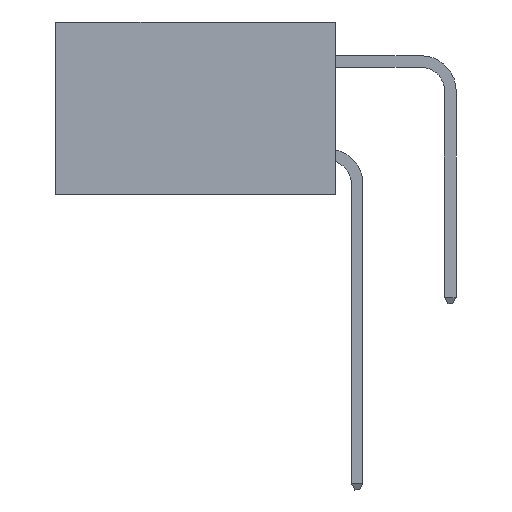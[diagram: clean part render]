
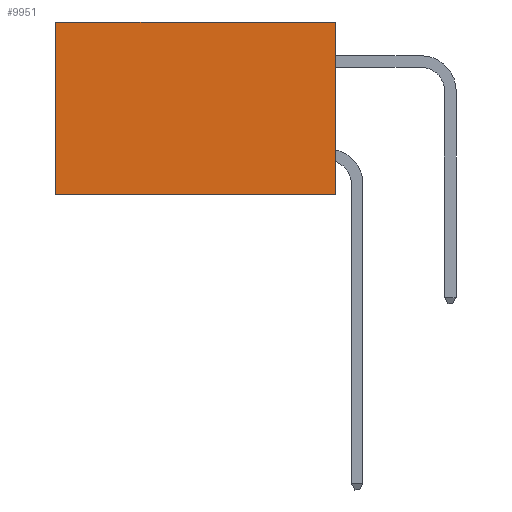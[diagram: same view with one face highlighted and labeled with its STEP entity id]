
A CAD part, left-side view. The second image highlights one B-rep face of the part: STEP entity #9951.
In plain terms, the highlighted planar face has unit normal (-1, 0, 0).
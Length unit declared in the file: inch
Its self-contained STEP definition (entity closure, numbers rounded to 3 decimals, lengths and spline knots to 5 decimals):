
#318 = VERTEX_POINT ( 'NONE', #5538 ) ;
#491 = EDGE_CURVE ( 'NONE', #8270, #14030, #4531, .T. ) ;
#507 = EDGE_CURVE ( 'NONE', #8270, #318, #3118, .T. ) ;
#1926 = CARTESIAN_POINT ( 'NONE',  ( 0.2875, 0., 0. ) ) ;
#3118 = LINE ( 'NONE', #14491, #26513 ) ;
#3299 = CARTESIAN_POINT ( 'NONE',  ( 0.2875, 0.6, -0.37 ) ) ;
#3526 = DIRECTION ( 'NONE',  ( 0., 0., -1. ) ) ;
#4531 = LINE ( 'NONE', #22821, #12783 ) ;
#5130 = LINE ( 'NONE', #15654, #13080 ) ;
#5538 = CARTESIAN_POINT ( 'NONE',  ( 0.2875, 0., -0.37 ) ) ;
#7276 = AXIS2_PLACEMENT_3D ( 'NONE', #1926, #15092, #8296 ) ;
#8270 = VERTEX_POINT ( 'NONE', #23688 ) ;
#8296 = DIRECTION ( 'NONE',  ( 0., 0., -1. ) ) ;
#8496 = PLANE ( 'NONE',  #7276 ) ;
#9399 = ORIENTED_EDGE ( 'NONE', *, *, #507, .F. ) ;
#9932 = EDGE_CURVE ( 'NONE', #318, #18418, #13407, .T. ) ;
#9951 = ADVANCED_FACE ( 'NONE', ( #11327 ), #8496, .F. ) ;
#11327 = FACE_OUTER_BOUND ( 'NONE', #23332, .T. ) ;
#11796 = DIRECTION ( 'NONE',  ( 0., 1., 0. ) ) ;
#12086 = ORIENTED_EDGE ( 'NONE', *, *, #21168, .T. ) ;
#12783 = VECTOR ( 'NONE', #11796, 39.37008 ) ;
#13080 = VECTOR ( 'NONE', #20025, 39.37008 ) ;
#13407 = LINE ( 'NONE', #26039, #23679 ) ;
#14030 = VERTEX_POINT ( 'NONE', #16364 ) ;
#14491 = CARTESIAN_POINT ( 'NONE',  ( 0.2875, 0., 0. ) ) ;
#15092 = DIRECTION ( 'NONE',  ( 1., 0., 0. ) ) ;
#15654 = CARTESIAN_POINT ( 'NONE',  ( 0.2875, 0.6, 0. ) ) ;
#16364 = CARTESIAN_POINT ( 'NONE',  ( 0.2875, 0.6, 0. ) ) ;
#18418 = VERTEX_POINT ( 'NONE', #3299 ) ;
#18636 = ORIENTED_EDGE ( 'NONE', *, *, #491, .T. ) ;
#20025 = DIRECTION ( 'NONE',  ( 0., 0., -1. ) ) ;
#21168 = EDGE_CURVE ( 'NONE', #14030, #18418, #5130, .T. ) ;
#22821 = CARTESIAN_POINT ( 'NONE',  ( 0.2875, 0., 0. ) ) ;
#23332 = EDGE_LOOP ( 'NONE', ( #12086, #27605, #9399, #18636 ) ) ;
#23679 = VECTOR ( 'NONE', #25850, 39.37008 ) ;
#23688 = CARTESIAN_POINT ( 'NONE',  ( 0.2875, 0., 0. ) ) ;
#25850 = DIRECTION ( 'NONE',  ( 0., 1., 0. ) ) ;
#26039 = CARTESIAN_POINT ( 'NONE',  ( 0.2875, 0., -0.37 ) ) ;
#26513 = VECTOR ( 'NONE', #3526, 39.37008 ) ;
#27605 = ORIENTED_EDGE ( 'NONE', *, *, #9932, .F. ) ;
